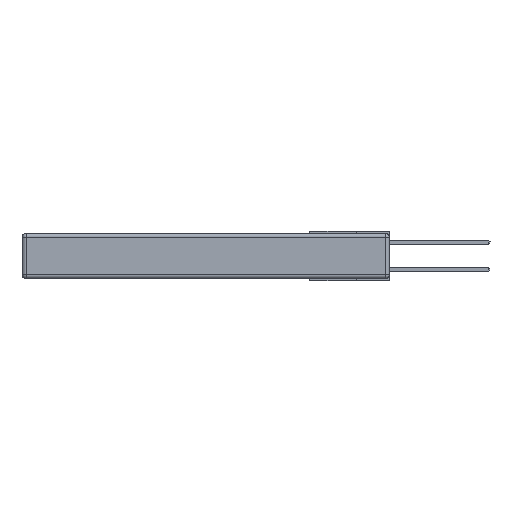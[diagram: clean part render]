
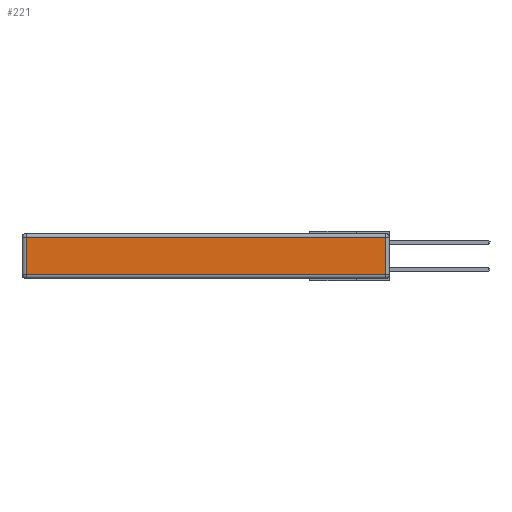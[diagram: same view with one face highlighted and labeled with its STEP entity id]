
A CAD part, left-side view. The second image highlights one B-rep face of the part: STEP entity #221.
In plain terms, the highlighted planar face has unit normal (-1, 0, 0).
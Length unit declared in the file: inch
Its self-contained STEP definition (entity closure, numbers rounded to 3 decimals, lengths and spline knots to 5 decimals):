
#221 = ADVANCED_FACE ( 'NONE', ( #9205 ), #20738, .T. ) ;
#748 = LINE ( 'NONE', #1415, #21167 ) ;
#939 = EDGE_CURVE ( 'NONE', #6233, #15249, #14547, .T. ) ;
#1415 = CARTESIAN_POINT ( 'NONE',  ( 0., 0.03, -0.343 ) ) ;
#1607 = LINE ( 'NONE', #14820, #2144 ) ;
#2144 = VECTOR ( 'NONE', #14895, 39.37008 ) ;
#2609 = LINE ( 'NONE', #18032, #11673 ) ;
#3820 = DIRECTION ( 'NONE',  ( 0., 0., 1. ) ) ;
#4007 = VERTEX_POINT ( 'NONE', #15899 ) ;
#5050 = VERTEX_POINT ( 'NONE', #13878 ) ;
#5385 = AXIS2_PLACEMENT_3D ( 'NONE', #8857, #12134, #3820 ) ;
#6233 = VERTEX_POINT ( 'NONE', #7502 ) ;
#7502 = CARTESIAN_POINT ( 'NONE',  ( 0., 2.72, -0.313 ) ) ;
#7868 = VECTOR ( 'NONE', #20208, 39.37008 ) ;
#8668 = EDGE_CURVE ( 'NONE', #4007, #6233, #1607, .T. ) ;
#8857 = CARTESIAN_POINT ( 'NONE',  ( 0., 0., -0.343 ) ) ;
#8910 = ORIENTED_EDGE ( 'NONE', *, *, #13714, .T. ) ;
#9205 = FACE_OUTER_BOUND ( 'NONE', #18851, .T. ) ;
#9272 = DIRECTION ( 'NONE',  ( 0., 1., 0. ) ) ;
#11612 = ORIENTED_EDGE ( 'NONE', *, *, #8668, .T. ) ;
#11673 = VECTOR ( 'NONE', #9272, 39.37008 ) ;
#11718 = DIRECTION ( 'NONE',  ( 0., 0., 1. ) ) ;
#12134 = DIRECTION ( 'NONE',  ( -1., 0., 0. ) ) ;
#13714 = EDGE_CURVE ( 'NONE', #15249, #5050, #748, .T. ) ;
#13878 = CARTESIAN_POINT ( 'NONE',  ( 0., 0.03, -0.03 ) ) ;
#14547 = LINE ( 'NONE', #20051, #7868 ) ;
#14820 = CARTESIAN_POINT ( 'NONE',  ( 0., 2.72, -0.343 ) ) ;
#14895 = DIRECTION ( 'NONE',  ( 0., 0., -1. ) ) ;
#15249 = VERTEX_POINT ( 'NONE', #20366 ) ;
#15560 = ORIENTED_EDGE ( 'NONE', *, *, #939, .T. ) ;
#15899 = CARTESIAN_POINT ( 'NONE',  ( 0., 2.72, -0.03 ) ) ;
#18032 = CARTESIAN_POINT ( 'NONE',  ( 0., 2.75, -0.03 ) ) ;
#18851 = EDGE_LOOP ( 'NONE', ( #15560, #8910, #22145, #11612 ) ) ;
#20051 = CARTESIAN_POINT ( 'NONE',  ( 0., 0., -0.313 ) ) ;
#20208 = DIRECTION ( 'NONE',  ( 0., -1., 0. ) ) ;
#20366 = CARTESIAN_POINT ( 'NONE',  ( 0., 0.03, -0.313 ) ) ;
#20387 = EDGE_CURVE ( 'NONE', #5050, #4007, #2609, .T. ) ;
#20738 = PLANE ( 'NONE',  #5385 ) ;
#21167 = VECTOR ( 'NONE', #11718, 39.37008 ) ;
#22145 = ORIENTED_EDGE ( 'NONE', *, *, #20387, .T. ) ;
